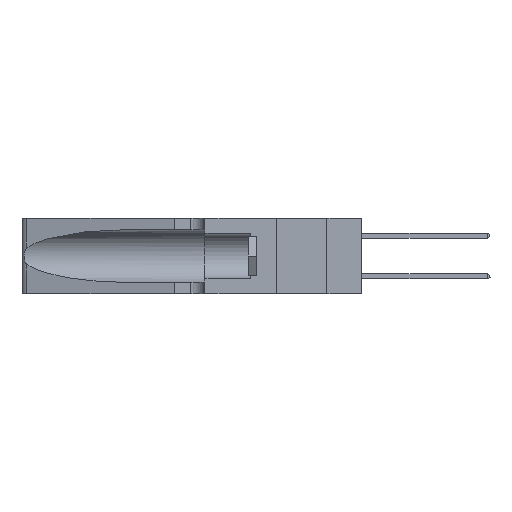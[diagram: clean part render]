
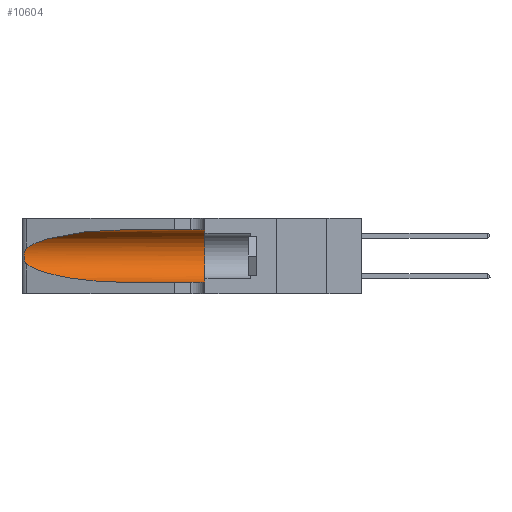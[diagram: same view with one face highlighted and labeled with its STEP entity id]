
A CAD part, left-side view. The second image highlights one B-rep face of the part: STEP entity #10604.
In plain terms, the highlighted cylindrical face has radius 3.308 mm (diameter 6.617 mm), a partial arc.
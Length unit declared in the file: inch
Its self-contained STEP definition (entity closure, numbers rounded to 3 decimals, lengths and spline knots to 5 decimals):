
#556 = CIRCLE ( 'NONE', #19594, 0.13025 ) ;
#620 = CARTESIAN_POINT ( 'NONE',  ( 0.25555, 1.22994, 0.2215 ) ) ;
#735 = CARTESIAN_POINT ( 'NONE',  ( 0.25854, 1.2359, 0.20912 ) ) ;
#827 = CARTESIAN_POINT ( 'NONE',  ( 0.25487, 1.22718, 0.14631 ) ) ;
#840 = CARTESIAN_POINT ( 'NONE',  ( 0.26075, 1.23896, 0.19203 ) ) ;
#3284 = CARTESIAN_POINT ( 'NONE',  ( 0.26017, 1.23833, 0.17102 ) ) ;
#3514 = CARTESIAN_POINT ( 'NONE',  ( 0.25487, 1.22718, 0.14631 ) ) ;
#3632 = ORIENTED_EDGE ( 'NONE', *, *, #7427, .F. ) ;
#3933 =( BOUNDED_CURVE ( )  B_SPLINE_CURVE ( 3, ( #17596, #31155, #15807, #26228 ),
 .UNSPECIFIED., .F., .T. ) 
 B_SPLINE_CURVE_WITH_KNOTS ( ( 4, 4 ),
 ( 3.44316, 4.71239 ),
 .UNSPECIFIED. ) 
 CURVE ( )  GEOMETRIC_REPRESENTATION_ITEM ( )  RATIONAL_B_SPLINE_CURVE ( ( 1., 0.87, 0.87, 1. ) ) 
 REPRESENTATION_ITEM ( '' )  );
#4352 = VERTEX_POINT ( 'NONE', #18288 ) ;
#4541 = LINE ( 'NONE', #11578, #29654 ) ;
#5847 = CARTESIAN_POINT ( 'NONE',  ( 0.25555, 1.22993, 0.14849 ) ) ;
#6611 = CARTESIAN_POINT ( 'NONE',  ( 0.25487, 1.22718, 0.22369 ) ) ;
#7427 = EDGE_CURVE ( 'NONE', #32218, #27231, #556, .T. ) ;
#7780 = DIRECTION ( 'NONE',  ( 0., -1., 0. ) ) ;
#8768 = EDGE_CURVE ( 'NONE', #4352, #27231, #9375, .T. ) ;
#9375 = LINE ( 'NONE', #24801, #22750 ) ;
#9546 = EDGE_CURVE ( 'NONE', #14202, #31293, #12145, .T. ) ;
#9651 = CARTESIAN_POINT ( 'NONE',  ( 0.18966, 0.96281, 0.31525 ) ) ;
#10604 = ADVANCED_FACE ( 'NONE', ( #26793 ), #18417, .F. ) ;
#11004 = CARTESIAN_POINT ( 'NONE',  ( 0.1305, 0.35, 0.05475 ) ) ;
#11216 = CARTESIAN_POINT ( 'NONE',  ( 0.1305, 0.35, 0.185 ) ) ;
#11456 = ORIENTED_EDGE ( 'NONE', *, *, #22884, .T. ) ;
#11578 = CARTESIAN_POINT ( 'NONE',  ( 0.1305, 1.61858, 0.31525 ) ) ;
#12114 = CARTESIAN_POINT ( 'NONE',  ( 0.1305, 0.72297, 0.31525 ) ) ;
#12145 =( BOUNDED_CURVE ( )  B_SPLINE_CURVE ( 3, ( #12114, #9651, #30838, #6611 ),
 .UNSPECIFIED., .F., .F. ) 
 B_SPLINE_CURVE_WITH_KNOTS ( ( 4, 4 ),
 ( 1.5708, 2.84003 ),
 .UNSPECIFIED. ) 
 CURVE ( )  GEOMETRIC_REPRESENTATION_ITEM ( )  RATIONAL_B_SPLINE_CURVE ( ( 1., 0.87, 0.87, 1. ) ) 
 REPRESENTATION_ITEM ( '' )  );
#12153 = EDGE_CURVE ( 'NONE', #14202, #32218, #4541, .T. ) ;
#13606 = CARTESIAN_POINT ( 'NONE',  ( 0.1305, 0.72297, 0.31525 ) ) ;
#13901 = CARTESIAN_POINT ( 'NONE',  ( 0.25789, 1.23486, 0.15765 ) ) ;
#14202 = VERTEX_POINT ( 'NONE', #13606 ) ;
#15139 = AXIS2_PLACEMENT_3D ( 'NONE', #26483, #7780, #31286 ) ;
#15207 = EDGE_LOOP ( 'NONE', ( #24768, #11456, #25318, #15397, #3632, #19011 ) ) ;
#15397 = ORIENTED_EDGE ( 'NONE', *, *, #8768, .T. ) ;
#15807 = CARTESIAN_POINT ( 'NONE',  ( 0.18966, 0.96281, 0.05475 ) ) ;
#16611 = DIRECTION ( 'NONE',  ( 0., 1., 0. ) ) ;
#16784 = EDGE_CURVE ( 'NONE', #27903, #4352, #3933, .T. ) ;
#16820 = CARTESIAN_POINT ( 'NONE',  ( 0.25787, 1.23484, 0.2124 ) ) ;
#16966 = CARTESIAN_POINT ( 'NONE',  ( 0.1305, 0.35, 0.31525 ) ) ;
#17596 = CARTESIAN_POINT ( 'NONE',  ( 0.25487, 1.22718, 0.14631 ) ) ;
#18288 = CARTESIAN_POINT ( 'NONE',  ( 0.1305, 0.72297, 0.05475 ) ) ;
#18417 = CYLINDRICAL_SURFACE ( 'NONE', #15139, 0.13025 ) ;
#19011 = ORIENTED_EDGE ( 'NONE', *, *, #12153, .F. ) ;
#19286 = CARTESIAN_POINT ( 'NONE',  ( 0.26075, 1.23896, 0.178 ) ) ;
#19534 = CARTESIAN_POINT ( 'NONE',  ( 0.25856, 1.23593, 0.16098 ) ) ;
#19594 = AXIS2_PLACEMENT_3D ( 'NONE', #11216, #16611, #30641 ) ;
#21394 = CARTESIAN_POINT ( 'NONE',  ( 0.25487, 1.22718, 0.22369 ) ) ;
#22091 = CARTESIAN_POINT ( 'NONE',  ( 0.25639, 1.23186, 0.15144 ) ) ;
#22210 = DIRECTION ( 'NONE',  ( 0., -1., 0. ) ) ;
#22750 = VECTOR ( 'NONE', #29952, 39.37008 ) ;
#22884 = EDGE_CURVE ( 'NONE', #31293, #27903, #25156, .T. ) ;
#24557 = CARTESIAN_POINT ( 'NONE',  ( 0.25639, 1.23184, 0.21858 ) ) ;
#24768 = ORIENTED_EDGE ( 'NONE', *, *, #9546, .T. ) ;
#24801 = CARTESIAN_POINT ( 'NONE',  ( 0.1305, 1.61858, 0.05475 ) ) ;
#25156 = B_SPLINE_CURVE_WITH_KNOTS ( 'NONE', 3,
 ( #21394, #620, #24557, #16820, #735, #32872, #840, #19286, #3284, #19534, #13901, #22091, #5847, #3514 ),
 .UNSPECIFIED., .F., .F.,
 ( 4, 2, 2, 2, 2, 2, 4 ),
 ( 0., 0.00027, 0.00053, 0.00107, 0.0016, 0.00187, 0.00214 ),
 .UNSPECIFIED. ) ;
#25318 = ORIENTED_EDGE ( 'NONE', *, *, #16784, .T. ) ;
#26228 = CARTESIAN_POINT ( 'NONE',  ( 0.1305, 0.72297, 0.05475 ) ) ;
#26483 = CARTESIAN_POINT ( 'NONE',  ( 0.1305, 1.61858, 0.185 ) ) ;
#26618 = CARTESIAN_POINT ( 'NONE',  ( 0.25487, 1.22718, 0.22369 ) ) ;
#26793 = FACE_OUTER_BOUND ( 'NONE', #15207, .T. ) ;
#27231 = VERTEX_POINT ( 'NONE', #11004 ) ;
#27903 = VERTEX_POINT ( 'NONE', #827 ) ;
#29654 = VECTOR ( 'NONE', #22210, 39.37008 ) ;
#29952 = DIRECTION ( 'NONE',  ( 0., -1., 0. ) ) ;
#30641 = DIRECTION ( 'NONE',  ( 0., 0., 1. ) ) ;
#30838 = CARTESIAN_POINT ( 'NONE',  ( 0.2373, 1.15595, 0.28018 ) ) ;
#31155 = CARTESIAN_POINT ( 'NONE',  ( 0.2373, 1.15595, 0.08982 ) ) ;
#31286 = DIRECTION ( 'NONE',  ( 0., 0., -1. ) ) ;
#31293 = VERTEX_POINT ( 'NONE', #26618 ) ;
#32218 = VERTEX_POINT ( 'NONE', #16966 ) ;
#32872 = CARTESIAN_POINT ( 'NONE',  ( 0.26018, 1.23835, 0.19895 ) ) ;
